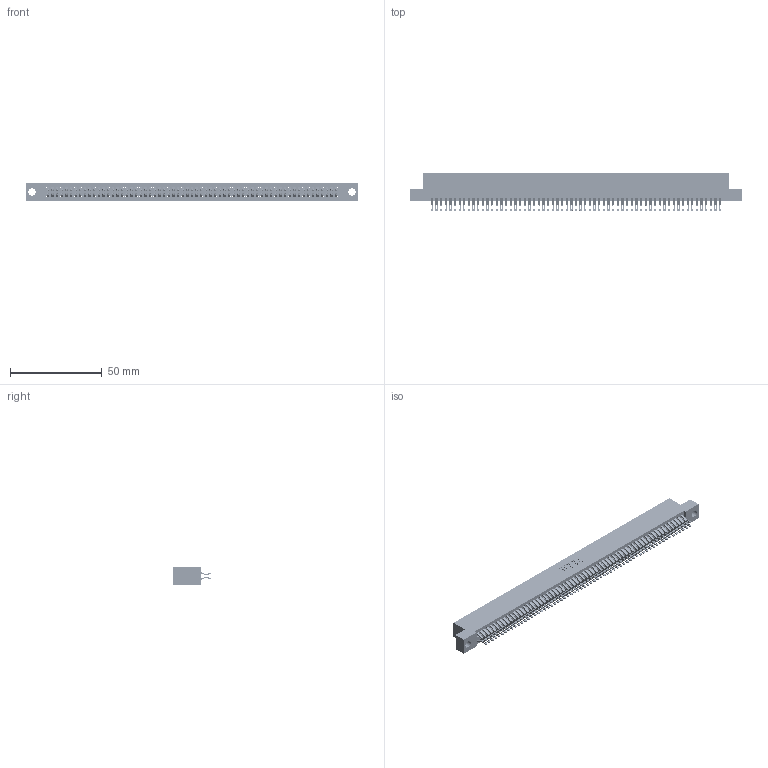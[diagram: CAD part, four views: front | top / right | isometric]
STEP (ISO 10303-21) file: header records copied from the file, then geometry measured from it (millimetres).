
FILE_DESCRIPTION (( 'STEP AP203' ), '1' );
FILE_NAME ('345-126-555-204.STEP', '2021-05-25T19:15:45', ( '' ), ( '' ), 'SwSTEP 2.0', 'SolidWorks 2020', '' );
FILE_SCHEMA (( 'CONFIG_CONTROL_DESIGN' ));
Length unit declared in the file: inch
Products named in the file (3): 345-126-555-204; 345 Part_Flush Mounting Lugs - 0.156 Dia-TI; 345-292-001_555 Tail
Assembly tree (127 placements, depth 2):
  345-126-555-204
    345 Part_Flush Mounting Lugs - 0.156 Dia-TI
    345-292-001_555 Tail  x126
Bounding box: 181.23 x 21.13 x 9.4 mm (x, y, z)
Volume: 18059.2 mm3; surface area: 28224 mm2
Topology: 127 solids, 127 shells, 7196 faces, 22679 edges, 15118 vertices
Faces by surface type: plane 4000, cylinder 3196
Entity records: 47349 total; most frequent: CARTESIAN_POINT 7956, ORIENTED_EDGE 7858, DIRECTION 6957, EDGE_CURVE 3929, LINE 3525, VECTOR 3525, VERTEX_POINT 2618, AXIS2_PLACEMENT_3D 1716
